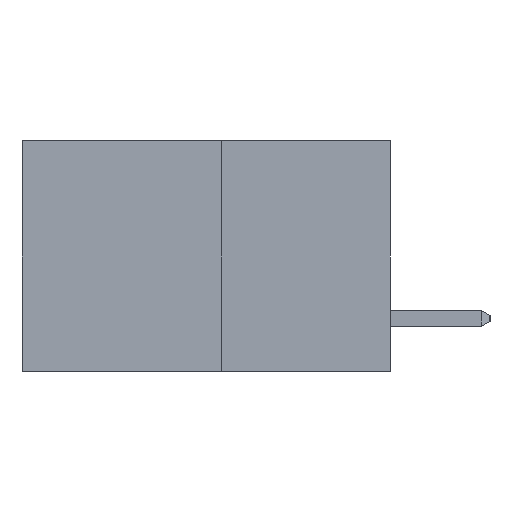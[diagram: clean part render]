
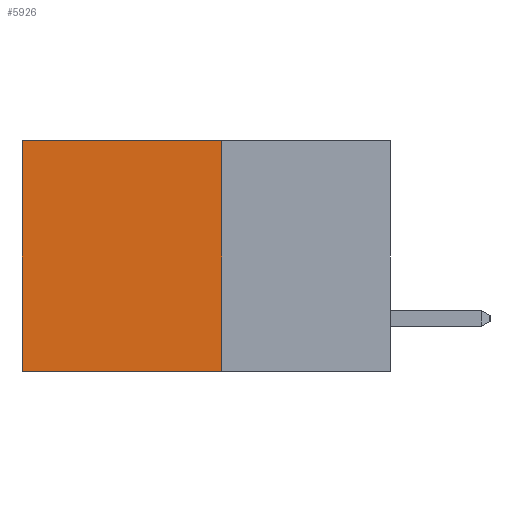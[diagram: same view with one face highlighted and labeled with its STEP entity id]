
A CAD part, left-side view. The second image highlights one B-rep face of the part: STEP entity #5926.
In plain terms, the highlighted planar face has unit normal (-1, 0, 0).
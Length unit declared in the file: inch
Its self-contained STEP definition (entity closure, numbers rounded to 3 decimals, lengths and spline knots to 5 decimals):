
#210 = EDGE_LOOP ( 'NONE', ( #1793, #7187, #7405, #3736 ) ) ;
#686 = CARTESIAN_POINT ( 'NONE',  ( 0.277, 0.27, 0. ) ) ;
#1018 = AXIS2_PLACEMENT_3D ( 'NONE', #6060, #2091, #6767 ) ;
#1175 = DIRECTION ( 'NONE',  ( 0., 1., 0. ) ) ;
#1751 = VERTEX_POINT ( 'NONE', #6058 ) ;
#1793 = ORIENTED_EDGE ( 'NONE', *, *, #5693, .T. ) ;
#2091 = DIRECTION ( 'NONE',  ( 1., 0., 0. ) ) ;
#2098 = EDGE_CURVE ( 'NONE', #4027, #1751, #8936, .T. ) ;
#2197 = CARTESIAN_POINT ( 'NONE',  ( 0.277, 0.27, -0.37 ) ) ;
#2416 = PLANE ( 'NONE',  #1018 ) ;
#2792 = DIRECTION ( 'NONE',  ( 0., 1., 0. ) ) ;
#2830 = EDGE_CURVE ( 'NONE', #4641, #4027, #4935, .T. ) ;
#3047 = VECTOR ( 'NONE', #6945, 39.37008 ) ;
#3167 = CARTESIAN_POINT ( 'NONE',  ( 0.277, 0.59, 0. ) ) ;
#3324 = DIRECTION ( 'NONE',  ( 0., 0., -1. ) ) ;
#3468 = LINE ( 'NONE', #4306, #6758 ) ;
#3736 = ORIENTED_EDGE ( 'NONE', *, *, #4112, .T. ) ;
#4027 = VERTEX_POINT ( 'NONE', #2197 ) ;
#4112 = EDGE_CURVE ( 'NONE', #4641, #7807, #3468, .T. ) ;
#4306 = CARTESIAN_POINT ( 'NONE',  ( 0.277, 0.27, 0. ) ) ;
#4641 = VERTEX_POINT ( 'NONE', #686 ) ;
#4935 = LINE ( 'NONE', #6882, #3047 ) ;
#5007 = FACE_OUTER_BOUND ( 'NONE', #210, .T. ) ;
#5693 = EDGE_CURVE ( 'NONE', #7807, #1751, #7349, .T. ) ;
#5926 = ADVANCED_FACE ( 'NONE', ( #5007 ), #2416, .F. ) ;
#6058 = CARTESIAN_POINT ( 'NONE',  ( 0.277, 0.59, -0.37 ) ) ;
#6060 = CARTESIAN_POINT ( 'NONE',  ( 0.277, 0.27, -0.37 ) ) ;
#6758 = VECTOR ( 'NONE', #2792, 39.37008 ) ;
#6767 = DIRECTION ( 'NONE',  ( 0., 0., -1. ) ) ;
#6882 = CARTESIAN_POINT ( 'NONE',  ( 0.277, 0.27, -0.37 ) ) ;
#6945 = DIRECTION ( 'NONE',  ( 0., 0., -1. ) ) ;
#7090 = CARTESIAN_POINT ( 'NONE',  ( 0.277, 0.27, -0.37 ) ) ;
#7187 = ORIENTED_EDGE ( 'NONE', *, *, #2098, .F. ) ;
#7293 = VECTOR ( 'NONE', #1175, 39.37008 ) ;
#7349 = LINE ( 'NONE', #8239, #8990 ) ;
#7405 = ORIENTED_EDGE ( 'NONE', *, *, #2830, .F. ) ;
#7807 = VERTEX_POINT ( 'NONE', #3167 ) ;
#8239 = CARTESIAN_POINT ( 'NONE',  ( 0.277, 0.59, -0.37 ) ) ;
#8936 = LINE ( 'NONE', #7090, #7293 ) ;
#8990 = VECTOR ( 'NONE', #3324, 39.37008 ) ;
